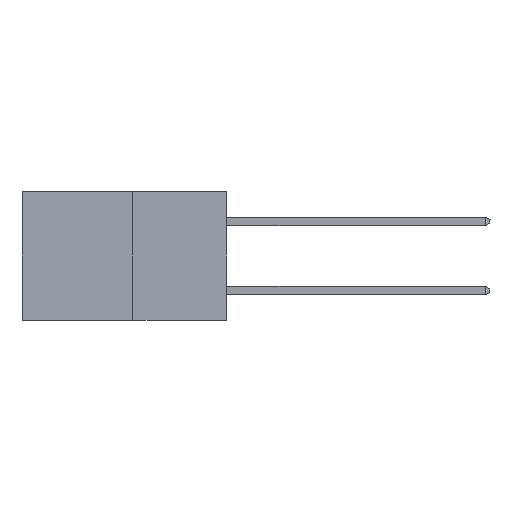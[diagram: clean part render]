
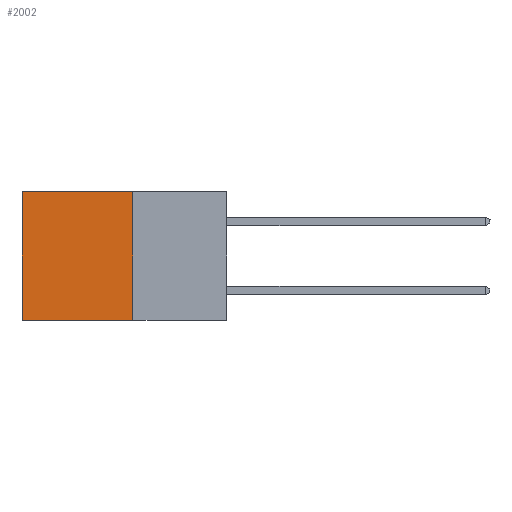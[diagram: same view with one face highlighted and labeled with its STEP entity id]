
A CAD part, left-side view. The second image highlights one B-rep face of the part: STEP entity #2002.
In plain terms, the highlighted planar face has unit normal (-1, 0, 0).
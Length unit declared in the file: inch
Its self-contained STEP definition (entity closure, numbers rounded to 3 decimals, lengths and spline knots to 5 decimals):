
#950 = DIRECTION ( 'NONE',  ( 0., 0., -1. ) ) ;
#1245 = ORIENTED_EDGE ( 'NONE', *, *, #8519, .F. ) ;
#1258 = DIRECTION ( 'NONE',  ( 0., 0., -1. ) ) ;
#1289 = VERTEX_POINT ( 'NONE', #3327 ) ;
#2002 = ADVANCED_FACE ( 'NONE', ( #6635 ), #9224, .F. ) ;
#2601 = LINE ( 'NONE', #10447, #8405 ) ;
#3041 = VERTEX_POINT ( 'NONE', #4016 ) ;
#3327 = CARTESIAN_POINT ( 'NONE',  ( 0.277, 0.27, 0. ) ) ;
#3480 = CARTESIAN_POINT ( 'NONE',  ( 0.277, 0.27, -0.37 ) ) ;
#4016 = CARTESIAN_POINT ( 'NONE',  ( 0.277, 0.59, -0.37 ) ) ;
#4269 = LINE ( 'NONE', #8327, #13347 ) ;
#4469 = ORIENTED_EDGE ( 'NONE', *, *, #10157, .F. ) ;
#5121 = EDGE_LOOP ( 'NONE', ( #7850, #4469, #1245, #13207 ) ) ;
#6457 = CARTESIAN_POINT ( 'NONE',  ( 0.277, 0.59, 0. ) ) ;
#6635 = FACE_OUTER_BOUND ( 'NONE', #5121, .T. ) ;
#6659 = VERTEX_POINT ( 'NONE', #8687 ) ;
#6754 = VERTEX_POINT ( 'NONE', #6457 ) ;
#6982 = CARTESIAN_POINT ( 'NONE',  ( 0.277, 0.27, -0.37 ) ) ;
#7263 = VECTOR ( 'NONE', #11967, 39.37008 ) ;
#7850 = ORIENTED_EDGE ( 'NONE', *, *, #10287, .T. ) ;
#8327 = CARTESIAN_POINT ( 'NONE',  ( 0.277, 0.59, -0.37 ) ) ;
#8405 = VECTOR ( 'NONE', #11558, 39.37008 ) ;
#8451 = LINE ( 'NONE', #6982, #14439 ) ;
#8519 = EDGE_CURVE ( 'NONE', #1289, #6659, #8451, .T. ) ;
#8687 = CARTESIAN_POINT ( 'NONE',  ( 0.277, 0.27, -0.37 ) ) ;
#9224 = PLANE ( 'NONE',  #10922 ) ;
#9356 = DIRECTION ( 'NONE',  ( 0., 0., -1. ) ) ;
#9573 = DIRECTION ( 'NONE',  ( 1., 0., 0. ) ) ;
#9662 = EDGE_CURVE ( 'NONE', #1289, #6754, #10386, .T. ) ;
#9722 = CARTESIAN_POINT ( 'NONE',  ( 0.277, 0.27, 0. ) ) ;
#10157 = EDGE_CURVE ( 'NONE', #6659, #3041, #2601, .T. ) ;
#10287 = EDGE_CURVE ( 'NONE', #6754, #3041, #4269, .T. ) ;
#10386 = LINE ( 'NONE', #9722, #7263 ) ;
#10447 = CARTESIAN_POINT ( 'NONE',  ( 0.277, 0.27, -0.37 ) ) ;
#10922 = AXIS2_PLACEMENT_3D ( 'NONE', #3480, #9573, #950 ) ;
#11558 = DIRECTION ( 'NONE',  ( 0., 1., 0. ) ) ;
#11967 = DIRECTION ( 'NONE',  ( 0., 1., 0. ) ) ;
#13207 = ORIENTED_EDGE ( 'NONE', *, *, #9662, .T. ) ;
#13347 = VECTOR ( 'NONE', #1258, 39.37008 ) ;
#14439 = VECTOR ( 'NONE', #9356, 39.37008 ) ;
